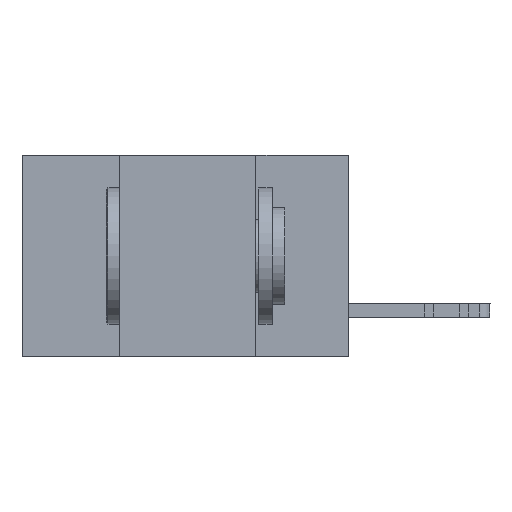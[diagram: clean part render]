
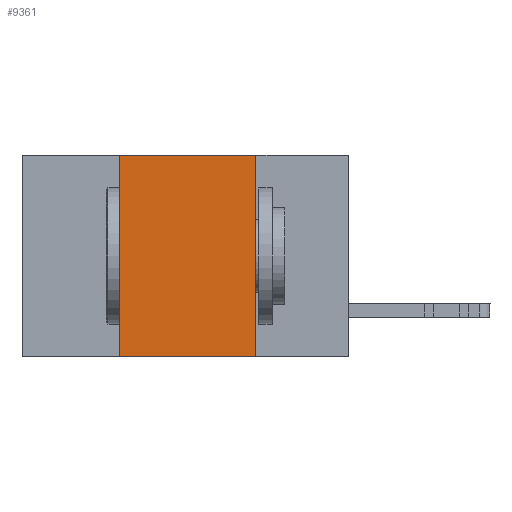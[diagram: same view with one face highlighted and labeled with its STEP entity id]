
A CAD part, left-side view. The second image highlights one B-rep face of the part: STEP entity #9361.
In plain terms, the highlighted planar face has unit normal (-1, 0, 0).
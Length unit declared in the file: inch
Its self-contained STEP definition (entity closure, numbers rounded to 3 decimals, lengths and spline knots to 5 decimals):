
#180 = LINE ( 'NONE', #10725, #18547 ) ;
#1635 = EDGE_CURVE ( 'NONE', #12248, #4416, #180, .T. ) ;
#2782 = DIRECTION ( 'NONE',  ( 0., 0., 1. ) ) ;
#4278 = CARTESIAN_POINT ( 'NONE',  ( 0., 0.6, 0. ) ) ;
#4416 = VERTEX_POINT ( 'NONE', #27213 ) ;
#5508 = VERTEX_POINT ( 'NONE', #11542 ) ;
#5885 = ORIENTED_EDGE ( 'NONE', *, *, #27649, .T. ) ;
#6298 = EDGE_CURVE ( 'NONE', #5508, #12248, #26668, .T. ) ;
#6904 = ORIENTED_EDGE ( 'NONE', *, *, #6298, .F. ) ;
#9361 = ADVANCED_FACE ( 'NONE', ( #20171 ), #23209, .F. ) ;
#10725 = CARTESIAN_POINT ( 'NONE',  ( 0., 0.17, 0. ) ) ;
#11513 = DIRECTION ( 'NONE',  ( 0., 0., -1. ) ) ;
#11542 = CARTESIAN_POINT ( 'NONE',  ( 0., 0.42, 0. ) ) ;
#11991 = DIRECTION ( 'NONE',  ( 0., 0., -1. ) ) ;
#12248 = VERTEX_POINT ( 'NONE', #18789 ) ;
#14292 = CARTESIAN_POINT ( 'NONE',  ( 0., 0.6, 0. ) ) ;
#14300 = DIRECTION ( 'NONE',  ( 0., -1., 0. ) ) ;
#14721 = CARTESIAN_POINT ( 'NONE',  ( 0., 0.42, 0. ) ) ;
#16772 = ORIENTED_EDGE ( 'NONE', *, *, #1635, .F. ) ;
#18384 = VERTEX_POINT ( 'NONE', #27854 ) ;
#18547 = VECTOR ( 'NONE', #11991, 39.37008 ) ;
#18789 = CARTESIAN_POINT ( 'NONE',  ( 0., 0.17, 0. ) ) ;
#20171 = FACE_OUTER_BOUND ( 'NONE', #25542, .T. ) ;
#20293 = AXIS2_PLACEMENT_3D ( 'NONE', #4278, #25677, #11513 ) ;
#20879 = LINE ( 'NONE', #28413, #27082 ) ;
#21211 = VECTOR ( 'NONE', #24063, 39.37008 ) ;
#22214 = ORIENTED_EDGE ( 'NONE', *, *, #29222, .F. ) ;
#23209 = PLANE ( 'NONE',  #20293 ) ;
#23669 = VECTOR ( 'NONE', #2782, 39.37008 ) ;
#24063 = DIRECTION ( 'NONE',  ( 0., -1., 0. ) ) ;
#25542 = EDGE_LOOP ( 'NONE', ( #16772, #6904, #22214, #5885 ) ) ;
#25677 = DIRECTION ( 'NONE',  ( 1., 0., 0. ) ) ;
#26668 = LINE ( 'NONE', #14292, #21211 ) ;
#27082 = VECTOR ( 'NONE', #14300, 39.37008 ) ;
#27213 = CARTESIAN_POINT ( 'NONE',  ( 0., 0.17, -0.37 ) ) ;
#27649 = EDGE_CURVE ( 'NONE', #18384, #4416, #20879, .T. ) ;
#27854 = CARTESIAN_POINT ( 'NONE',  ( 0., 0.42, -0.37 ) ) ;
#28413 = CARTESIAN_POINT ( 'NONE',  ( 0., 0.6, -0.37 ) ) ;
#29222 = EDGE_CURVE ( 'NONE', #18384, #5508, #30603, .T. ) ;
#30603 = LINE ( 'NONE', #14721, #23669 ) ;
